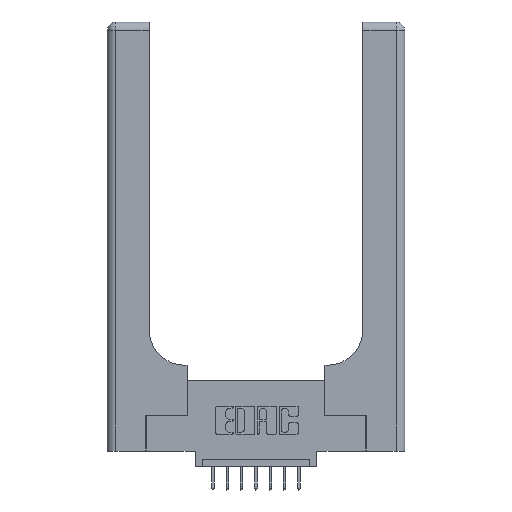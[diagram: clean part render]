
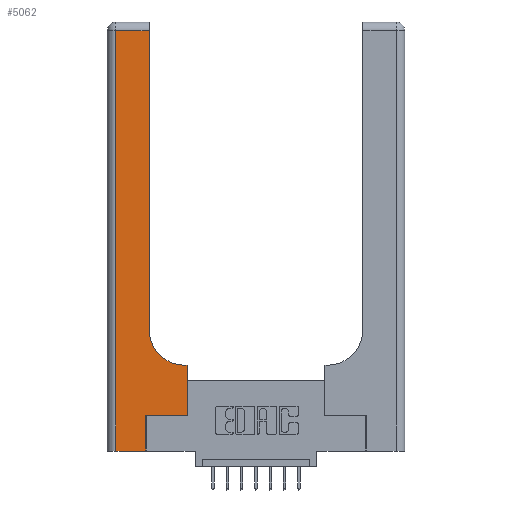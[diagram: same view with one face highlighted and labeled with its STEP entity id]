
A CAD part, top view. The second image highlights one B-rep face of the part: STEP entity #5062.
In plain terms, the highlighted planar face has unit normal (0, 0, 1).
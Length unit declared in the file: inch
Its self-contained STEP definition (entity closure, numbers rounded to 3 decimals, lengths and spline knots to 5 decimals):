
#213 = DIRECTION ( 'NONE',  ( 0., 1., 0. ) ) ;
#274 = VERTEX_POINT ( 'NONE', #14318 ) ;
#319 = VECTOR ( 'NONE', #213, 39.37008 ) ;
#449 = CARTESIAN_POINT ( 'NONE',  ( 0., 0., 0.37 ) ) ;
#562 = VERTEX_POINT ( 'NONE', #9154 ) ;
#742 = ORIENTED_EDGE ( 'NONE', *, *, #11502, .T. ) ;
#835 = EDGE_CURVE ( 'NONE', #6010, #8734, #12056, .T. ) ;
#950 = ORIENTED_EDGE ( 'NONE', *, *, #4386, .T. ) ;
#982 = LINE ( 'NONE', #4291, #15275 ) ;
#1388 = EDGE_CURVE ( 'NONE', #5213, #9682, #12226, .T. ) ;
#1809 = CARTESIAN_POINT ( 'NONE',  ( 0., 2.94, 0.37 ) ) ;
#2004 = LINE ( 'NONE', #5778, #9015 ) ;
#2156 = CARTESIAN_POINT ( 'NONE',  ( 0.269, 0.25, 0.37 ) ) ;
#2238 = CARTESIAN_POINT ( 'NONE',  ( 0., 3., 0.37 ) ) ;
#2343 = DIRECTION ( 'NONE',  ( 1., 0., 0. ) ) ;
#2358 = LINE ( 'NONE', #5989, #319 ) ;
#2384 = LINE ( 'NONE', #1809, #2553 ) ;
#2553 = VECTOR ( 'NONE', #12697, 39.37008 ) ;
#2642 = FACE_OUTER_BOUND ( 'NONE', #5050, .T. ) ;
#2658 = CARTESIAN_POINT ( 'NONE',  ( 0.06, 2.94, 0.37 ) ) ;
#2702 = CARTESIAN_POINT ( 'NONE',  ( 0.5415, 0.6, 0.37 ) ) ;
#3086 = VECTOR ( 'NONE', #5438, 39.37008 ) ;
#3172 = ORIENTED_EDGE ( 'NONE', *, *, #8105, .T. ) ;
#3188 = EDGE_CURVE ( 'NONE', #9682, #12936, #3978, .T. ) ;
#3787 = ORIENTED_EDGE ( 'NONE', *, *, #5004, .T. ) ;
#3978 = LINE ( 'NONE', #10939, #3086 ) ;
#4107 = VERTEX_POINT ( 'NONE', #7735 ) ;
#4291 = CARTESIAN_POINT ( 'NONE',  ( 0.2915, 3., 0.37 ) ) ;
#4342 = DIRECTION ( 'NONE',  ( 0., 1., 0. ) ) ;
#4386 = EDGE_CURVE ( 'NONE', #8734, #562, #5985, .T. ) ;
#4702 = CARTESIAN_POINT ( 'NONE',  ( 0.06, 0., 0.37 ) ) ;
#5004 = EDGE_CURVE ( 'NONE', #8402, #4107, #13053, .T. ) ;
#5050 = EDGE_LOOP ( 'NONE', ( #10067, #12745, #10290, #950, #742, #11094, #12263, #3172, #3787 ) ) ;
#5062 = ADVANCED_FACE ( 'NONE', ( #2642 ), #10552, .F. ) ;
#5213 = VERTEX_POINT ( 'NONE', #2156 ) ;
#5438 = DIRECTION ( 'NONE',  ( 0., 1., 0. ) ) ;
#5733 = DIRECTION ( 'NONE',  ( -1., 0., 0. ) ) ;
#5778 = CARTESIAN_POINT ( 'NONE',  ( 0.2915, 0.6, 0.37 ) ) ;
#5985 = LINE ( 'NONE', #449, #8757 ) ;
#5989 = CARTESIAN_POINT ( 'NONE',  ( 0.269, 0., 0.37 ) ) ;
#6010 = VERTEX_POINT ( 'NONE', #2658 ) ;
#6710 = CARTESIAN_POINT ( 'NONE',  ( 0.5585, 0.6, 0.37 ) ) ;
#6752 = DIRECTION ( 'NONE',  ( 0., -1., 0. ) ) ;
#7613 = DIRECTION ( 'NONE',  ( 1., 0., 0. ) ) ;
#7735 = CARTESIAN_POINT ( 'NONE',  ( 0.2915, 0.85, 0.37 ) ) ;
#7780 = CARTESIAN_POINT ( 'NONE',  ( 0.269, 0.25, 0.37 ) ) ;
#7813 = EDGE_CURVE ( 'NONE', #274, #6010, #2384, .T. ) ;
#8105 = EDGE_CURVE ( 'NONE', #12936, #8402, #2004, .T. ) ;
#8402 = VERTEX_POINT ( 'NONE', #2702 ) ;
#8734 = VERTEX_POINT ( 'NONE', #4702 ) ;
#8757 = VECTOR ( 'NONE', #7613, 39.37008 ) ;
#8961 = CARTESIAN_POINT ( 'NONE',  ( 0.5585, 0.25, 0.37 ) ) ;
#9000 = DIRECTION ( 'NONE',  ( -1., 0., 0. ) ) ;
#9015 = VECTOR ( 'NONE', #9000, 39.37008 ) ;
#9154 = CARTESIAN_POINT ( 'NONE',  ( 0.269, 0., 0.37 ) ) ;
#9682 = VERTEX_POINT ( 'NONE', #8961 ) ;
#10007 = AXIS2_PLACEMENT_3D ( 'NONE', #2238, #12870, #5733 ) ;
#10067 = ORIENTED_EDGE ( 'NONE', *, *, #15342, .T. ) ;
#10290 = ORIENTED_EDGE ( 'NONE', *, *, #835, .T. ) ;
#10449 = DIRECTION ( 'NONE',  ( 0., 0., -1. ) ) ;
#10522 = VECTOR ( 'NONE', #12642, 39.37008 ) ;
#10552 = PLANE ( 'NONE',  #10007 ) ;
#10618 = AXIS2_PLACEMENT_3D ( 'NONE', #13074, #10449, #2343 ) ;
#10939 = CARTESIAN_POINT ( 'NONE',  ( 0.5585, 0.25, 0.37 ) ) ;
#11094 = ORIENTED_EDGE ( 'NONE', *, *, #1388, .T. ) ;
#11502 = EDGE_CURVE ( 'NONE', #562, #5213, #2358, .T. ) ;
#11850 = VECTOR ( 'NONE', #6752, 39.37008 ) ;
#12056 = LINE ( 'NONE', #13886, #11850 ) ;
#12226 = LINE ( 'NONE', #7780, #10522 ) ;
#12263 = ORIENTED_EDGE ( 'NONE', *, *, #3188, .T. ) ;
#12642 = DIRECTION ( 'NONE',  ( 1., 0., 0. ) ) ;
#12697 = DIRECTION ( 'NONE',  ( -1., 0., 0. ) ) ;
#12745 = ORIENTED_EDGE ( 'NONE', *, *, #7813, .T. ) ;
#12870 = DIRECTION ( 'NONE',  ( 0., 0., -1. ) ) ;
#12936 = VERTEX_POINT ( 'NONE', #6710 ) ;
#13053 = CIRCLE ( 'NONE', #10618, 0.25 ) ;
#13074 = CARTESIAN_POINT ( 'NONE',  ( 0.5415, 0.85, 0.37 ) ) ;
#13886 = CARTESIAN_POINT ( 'NONE',  ( 0.06, 3., 0.37 ) ) ;
#14318 = CARTESIAN_POINT ( 'NONE',  ( 0.2915, 2.94, 0.37 ) ) ;
#15275 = VECTOR ( 'NONE', #4342, 39.37008 ) ;
#15342 = EDGE_CURVE ( 'NONE', #4107, #274, #982, .T. ) ;
